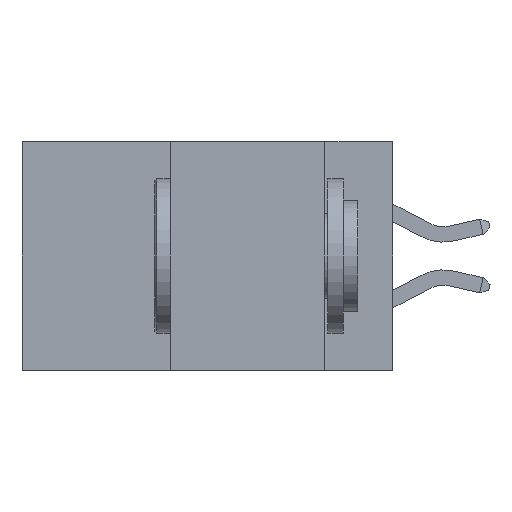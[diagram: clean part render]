
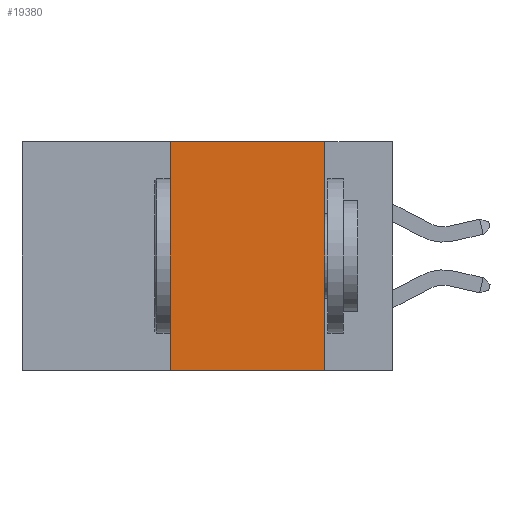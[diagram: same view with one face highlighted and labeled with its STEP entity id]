
A CAD part, left-side view. The second image highlights one B-rep face of the part: STEP entity #19380.
In plain terms, the highlighted planar face has unit normal (-1, 0, 0).
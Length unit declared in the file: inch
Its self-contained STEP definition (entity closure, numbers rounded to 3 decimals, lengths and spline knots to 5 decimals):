
#366 = CARTESIAN_POINT ( 'NONE',  ( 0., 0.11, 0. ) ) ;
#472 = CARTESIAN_POINT ( 'NONE',  ( 0., 0.11, 0. ) ) ;
#584 = LINE ( 'NONE', #14871, #1609 ) ;
#1007 = VERTEX_POINT ( 'NONE', #366 ) ;
#1609 = VECTOR ( 'NONE', #6820, 39.37008 ) ;
#3828 = ORIENTED_EDGE ( 'NONE', *, *, #17384, .T. ) ;
#4491 = LINE ( 'NONE', #15790, #20704 ) ;
#5187 = EDGE_CURVE ( 'NONE', #7132, #9064, #20571, .T. ) ;
#6820 = DIRECTION ( 'NONE',  ( 0., -1., 0. ) ) ;
#7132 = VERTEX_POINT ( 'NONE', #18916 ) ;
#7165 = DIRECTION ( 'NONE',  ( 1., 0., 0. ) ) ;
#7532 = EDGE_LOOP ( 'NONE', ( #14730, #19266, #13877, #3828 ) ) ;
#7883 = FACE_OUTER_BOUND ( 'NONE', #7532, .T. ) ;
#8378 = CARTESIAN_POINT ( 'NONE',  ( 0., 0.36, 0. ) ) ;
#9064 = VERTEX_POINT ( 'NONE', #10885 ) ;
#9862 = VECTOR ( 'NONE', #18218, 39.37008 ) ;
#10673 = CARTESIAN_POINT ( 'NONE',  ( 0., 0.11, -0.37 ) ) ;
#10885 = CARTESIAN_POINT ( 'NONE',  ( 0., 0.36, 0. ) ) ;
#11058 = DIRECTION ( 'NONE',  ( 0., -1., 0. ) ) ;
#12578 = VERTEX_POINT ( 'NONE', #10673 ) ;
#13403 = DIRECTION ( 'NONE',  ( 0., 0., 1. ) ) ;
#13877 = ORIENTED_EDGE ( 'NONE', *, *, #5187, .F. ) ;
#14730 = ORIENTED_EDGE ( 'NONE', *, *, #15545, .F. ) ;
#14871 = CARTESIAN_POINT ( 'NONE',  ( 0., 0.6, -0.37 ) ) ;
#15205 = AXIS2_PLACEMENT_3D ( 'NONE', #16627, #7165, #20013 ) ;
#15545 = EDGE_CURVE ( 'NONE', #1007, #12578, #18443, .T. ) ;
#15790 = CARTESIAN_POINT ( 'NONE',  ( 0., 0.6, 0. ) ) ;
#16036 = VECTOR ( 'NONE', #13403, 39.37008 ) ;
#16627 = CARTESIAN_POINT ( 'NONE',  ( 0., 0.6, 0. ) ) ;
#17384 = EDGE_CURVE ( 'NONE', #7132, #12578, #584, .T. ) ;
#18218 = DIRECTION ( 'NONE',  ( 0., 0., -1. ) ) ;
#18443 = LINE ( 'NONE', #472, #9862 ) ;
#18916 = CARTESIAN_POINT ( 'NONE',  ( 0., 0.36, -0.37 ) ) ;
#19266 = ORIENTED_EDGE ( 'NONE', *, *, #19758, .F. ) ;
#19380 = ADVANCED_FACE ( 'NONE', ( #7883 ), #19527, .F. ) ;
#19527 = PLANE ( 'NONE',  #15205 ) ;
#19758 = EDGE_CURVE ( 'NONE', #9064, #1007, #4491, .T. ) ;
#20013 = DIRECTION ( 'NONE',  ( 0., 0., -1. ) ) ;
#20571 = LINE ( 'NONE', #8378, #16036 ) ;
#20704 = VECTOR ( 'NONE', #11058, 39.37008 ) ;
